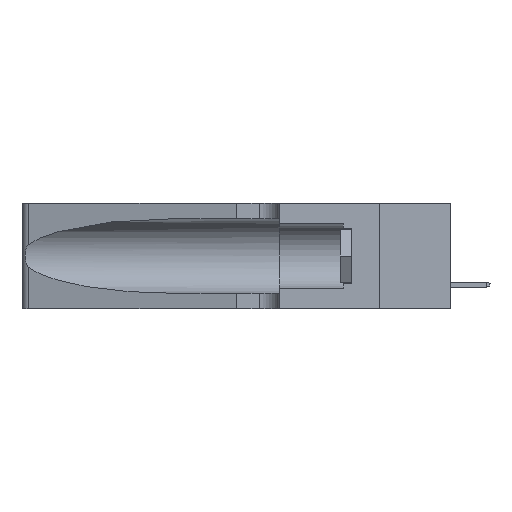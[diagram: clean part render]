
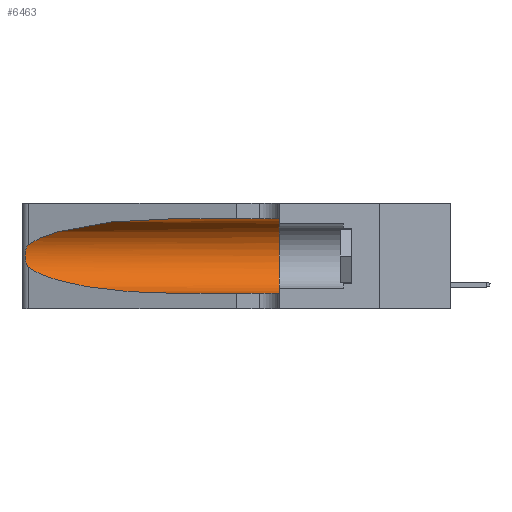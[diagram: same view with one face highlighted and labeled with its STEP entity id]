
A CAD part, left-side view. The second image highlights one B-rep face of the part: STEP entity #6463.
In plain terms, the highlighted cylindrical face has radius 3.308 mm (diameter 6.617 mm), a partial arc.
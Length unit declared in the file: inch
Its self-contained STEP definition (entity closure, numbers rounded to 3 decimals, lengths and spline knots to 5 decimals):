
#903 = DIRECTION ( 'NONE',  ( 0., 1., 0. ) ) ;
#1134 = EDGE_CURVE ( 'NONE', #17578, #11239, #17042, .T. ) ;
#1275 = EDGE_CURVE ( 'NONE', #18965, #18493, #32273, .T. ) ;
#1770 = CARTESIAN_POINT ( 'NONE',  ( 0.25487, 1.22718, 0.22369 ) ) ;
#1851 = CARTESIAN_POINT ( 'NONE',  ( 0.1305, 0.35, 0.31525 ) ) ;
#2432 = ORIENTED_EDGE ( 'NONE', *, *, #16415, .T. ) ;
#4635 = CARTESIAN_POINT ( 'NONE',  ( 0.25854, 1.2359, 0.20912 ) ) ;
#4796 = CARTESIAN_POINT ( 'NONE',  ( 0.25639, 1.23186, 0.15144 ) ) ;
#4975 = CARTESIAN_POINT ( 'NONE',  ( 0.25487, 1.22718, 0.14631 ) ) ;
#5603 = ORIENTED_EDGE ( 'NONE', *, *, #8245, .T. ) ;
#6463 = ADVANCED_FACE ( 'NONE', ( #12200 ), #11673, .F. ) ;
#7130 = CARTESIAN_POINT ( 'NONE',  ( 0.1305, 0.72297, 0.31525 ) ) ;
#7482 = CARTESIAN_POINT ( 'NONE',  ( 0.26075, 1.23896, 0.19203 ) ) ;
#8245 = EDGE_CURVE ( 'NONE', #18493, #17578, #8848, .T. ) ;
#8343 = VERTEX_POINT ( 'NONE', #1851 ) ;
#8640 = ORIENTED_EDGE ( 'NONE', *, *, #1275, .T. ) ;
#8848 =( BOUNDED_CURVE ( )  B_SPLINE_CURVE ( 3, ( #18703, #26717, #13200, #31710 ),
 .UNSPECIFIED., .F., .F. ) 
 B_SPLINE_CURVE_WITH_KNOTS ( ( 4, 4 ),
 ( 3.44316, 4.71239 ),
 .UNSPECIFIED. ) 
 CURVE ( )  GEOMETRIC_REPRESENTATION_ITEM ( )  RATIONAL_B_SPLINE_CURVE ( ( 1., 0.87, 0.87, 1. ) ) 
 REPRESENTATION_ITEM ( '' )  );
#8924 = EDGE_CURVE ( 'NONE', #9302, #8343, #11032, .T. ) ;
#9082 = DIRECTION ( 'NONE',  ( 0., -1., 0. ) ) ;
#9302 = VERTEX_POINT ( 'NONE', #7130 ) ;
#9786 = CARTESIAN_POINT ( 'NONE',  ( 0.25555, 1.22993, 0.14849 ) ) ;
#10199 = AXIS2_PLACEMENT_3D ( 'NONE', #14843, #19818, #28375 ) ;
#10463 = EDGE_LOOP ( 'NONE', ( #2432, #8640, #5603, #32684, #15439, #33175 ) ) ;
#10918 =( BOUNDED_CURVE ( )  B_SPLINE_CURVE ( 3, ( #20524, #29232, #18033, #20871 ),
 .UNSPECIFIED., .F., .F. ) 
 B_SPLINE_CURVE_WITH_KNOTS ( ( 4, 4 ),
 ( 1.5708, 2.84003 ),
 .UNSPECIFIED. ) 
 CURVE ( )  GEOMETRIC_REPRESENTATION_ITEM ( )  RATIONAL_B_SPLINE_CURVE ( ( 1., 0.87, 0.87, 1. ) ) 
 REPRESENTATION_ITEM ( '' )  );
#11025 = VECTOR ( 'NONE', #9082, 39.37008 ) ;
#11032 = LINE ( 'NONE', #24686, #32613 ) ;
#11209 = DIRECTION ( 'NONE',  ( 0., -1., 0. ) ) ;
#11239 = VERTEX_POINT ( 'NONE', #15908 ) ;
#11673 = CYLINDRICAL_SURFACE ( 'NONE', #10199, 0.13025 ) ;
#11742 = DIRECTION ( 'NONE',  ( 0., 0., 1. ) ) ;
#12200 = FACE_OUTER_BOUND ( 'NONE', #10463, .T. ) ;
#12453 = EDGE_CURVE ( 'NONE', #8343, #11239, #25383, .T. ) ;
#13200 = CARTESIAN_POINT ( 'NONE',  ( 0.18966, 0.96281, 0.05475 ) ) ;
#14843 = CARTESIAN_POINT ( 'NONE',  ( 0.1305, 1.61858, 0.185 ) ) ;
#15439 = ORIENTED_EDGE ( 'NONE', *, *, #12453, .F. ) ;
#15908 = CARTESIAN_POINT ( 'NONE',  ( 0.1305, 0.35, 0.05475 ) ) ;
#16415 = EDGE_CURVE ( 'NONE', #9302, #18965, #10918, .T. ) ;
#17042 = LINE ( 'NONE', #27897, #11025 ) ;
#17578 = VERTEX_POINT ( 'NONE', #24514 ) ;
#18033 = CARTESIAN_POINT ( 'NONE',  ( 0.2373, 1.15595, 0.28018 ) ) ;
#18439 = CARTESIAN_POINT ( 'NONE',  ( 0.25555, 1.22994, 0.2215 ) ) ;
#18493 = VERTEX_POINT ( 'NONE', #25246 ) ;
#18703 = CARTESIAN_POINT ( 'NONE',  ( 0.25487, 1.22718, 0.14631 ) ) ;
#18965 = VERTEX_POINT ( 'NONE', #19875 ) ;
#19818 = DIRECTION ( 'NONE',  ( 0., -1., 0. ) ) ;
#19875 = CARTESIAN_POINT ( 'NONE',  ( 0.25487, 1.22718, 0.22369 ) ) ;
#20524 = CARTESIAN_POINT ( 'NONE',  ( 0.1305, 0.72297, 0.31525 ) ) ;
#20871 = CARTESIAN_POINT ( 'NONE',  ( 0.25487, 1.22718, 0.22369 ) ) ;
#21280 = CARTESIAN_POINT ( 'NONE',  ( 0.25789, 1.23486, 0.15765 ) ) ;
#21995 = AXIS2_PLACEMENT_3D ( 'NONE', #25224, #903, #11742 ) ;
#24514 = CARTESIAN_POINT ( 'NONE',  ( 0.1305, 0.72297, 0.05475 ) ) ;
#24686 = CARTESIAN_POINT ( 'NONE',  ( 0.1305, 1.61858, 0.31525 ) ) ;
#25224 = CARTESIAN_POINT ( 'NONE',  ( 0.1305, 0.35, 0.185 ) ) ;
#25246 = CARTESIAN_POINT ( 'NONE',  ( 0.25487, 1.22718, 0.14631 ) ) ;
#25383 = CIRCLE ( 'NONE', #21995, 0.13025 ) ;
#26456 = CARTESIAN_POINT ( 'NONE',  ( 0.25639, 1.23184, 0.21858 ) ) ;
#26717 = CARTESIAN_POINT ( 'NONE',  ( 0.2373, 1.15595, 0.08982 ) ) ;
#27897 = CARTESIAN_POINT ( 'NONE',  ( 0.1305, 1.61858, 0.05475 ) ) ;
#28375 = DIRECTION ( 'NONE',  ( 0., 0., -1. ) ) ;
#28784 = CARTESIAN_POINT ( 'NONE',  ( 0.26017, 1.23833, 0.17102 ) ) ;
#29232 = CARTESIAN_POINT ( 'NONE',  ( 0.18966, 0.96281, 0.31525 ) ) ;
#29484 = CARTESIAN_POINT ( 'NONE',  ( 0.26018, 1.23835, 0.19895 ) ) ;
#31443 = CARTESIAN_POINT ( 'NONE',  ( 0.26075, 1.23896, 0.178 ) ) ;
#31710 = CARTESIAN_POINT ( 'NONE',  ( 0.1305, 0.72297, 0.05475 ) ) ;
#32273 = B_SPLINE_CURVE_WITH_KNOTS ( 'NONE', 3,
 ( #1770, #18439, #26456, #34803, #4635, #29484, #7482, #31443, #28784, #34106, #21280, #4796, #9786, #4975 ),
 .UNSPECIFIED., .F., .F.,
 ( 4, 2, 2, 2, 2, 2, 4 ),
 ( 0., 0.00027, 0.00053, 0.00107, 0.0016, 0.00187, 0.00214 ),
 .UNSPECIFIED. ) ;
#32613 = VECTOR ( 'NONE', #11209, 39.37008 ) ;
#32684 = ORIENTED_EDGE ( 'NONE', *, *, #1134, .T. ) ;
#33175 = ORIENTED_EDGE ( 'NONE', *, *, #8924, .F. ) ;
#34106 = CARTESIAN_POINT ( 'NONE',  ( 0.25856, 1.23593, 0.16098 ) ) ;
#34803 = CARTESIAN_POINT ( 'NONE',  ( 0.25787, 1.23484, 0.2124 ) ) ;
